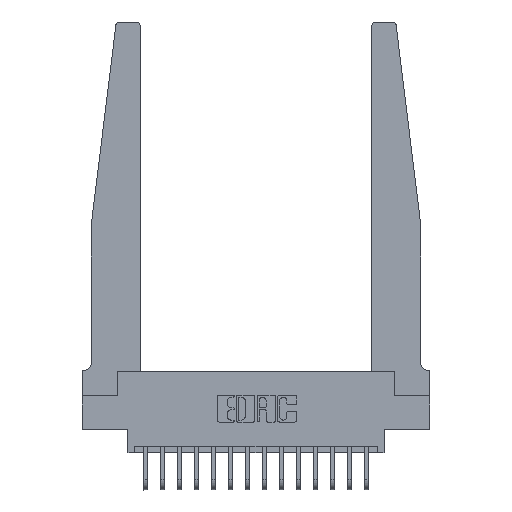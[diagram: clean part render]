
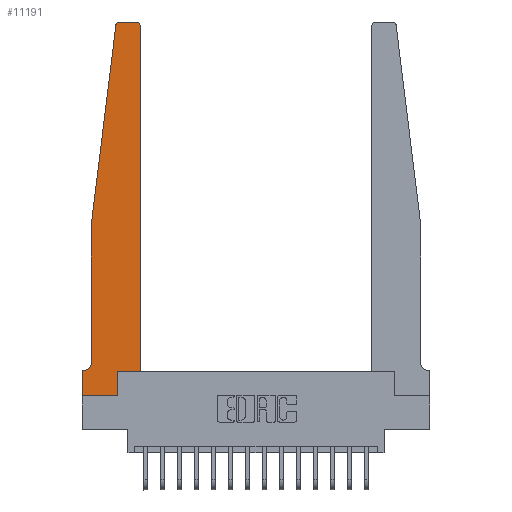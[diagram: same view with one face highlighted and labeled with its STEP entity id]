
A CAD part, top view. The second image highlights one B-rep face of the part: STEP entity #11191.
In plain terms, the highlighted planar face has unit normal (0, 0, 1).
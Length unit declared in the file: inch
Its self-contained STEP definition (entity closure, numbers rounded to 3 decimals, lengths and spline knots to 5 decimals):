
#123 = DIRECTION ( 'NONE',  ( 1., 0., 0. ) ) ;
#239 = CARTESIAN_POINT ( 'NONE',  ( 0.065, 0.2375, 0.37 ) ) ;
#549 = DIRECTION ( 'NONE',  ( -1., 0., 0. ) ) ;
#646 = DIRECTION ( 'NONE',  ( 0., 1., 0. ) ) ;
#913 = CARTESIAN_POINT ( 'NONE',  ( 0.425, 0.18, 0.37 ) ) ;
#951 = VERTEX_POINT ( 'NONE', #15004 ) ;
#1032 = DIRECTION ( 'NONE',  ( 0., 0., 1. ) ) ;
#1217 = PLANE ( 'NONE',  #14384 ) ;
#1465 = LINE ( 'NONE', #5619, #2724 ) ;
#1819 = DIRECTION ( 'NONE',  ( 0., -1., 0. ) ) ;
#1885 = VERTEX_POINT ( 'NONE', #15846 ) ;
#2092 = LINE ( 'NONE', #17278, #6125 ) ;
#2199 = EDGE_CURVE ( 'NONE', #13390, #1885, #1465, .T. ) ;
#2627 = VECTOR ( 'NONE', #4914, 39.37008 ) ;
#2724 = VECTOR ( 'NONE', #16654, 39.37008 ) ;
#2831 = DIRECTION ( 'NONE',  ( 0., 0., 1. ) ) ;
#2866 = VERTEX_POINT ( 'NONE', #12780 ) ;
#3019 = VERTEX_POINT ( 'NONE', #13405 ) ;
#3581 = ORIENTED_EDGE ( 'NONE', *, *, #2199, .T. ) ;
#3646 = VERTEX_POINT ( 'NONE', #12553 ) ;
#3770 = CARTESIAN_POINT ( 'NONE',  ( 0.065, 1.25, 0.37 ) ) ;
#3796 = EDGE_CURVE ( 'NONE', #3646, #10851, #15999, .T. ) ;
#3837 = CARTESIAN_POINT ( 'NONE',  ( 0., 0.1875, 0.37 ) ) ;
#3959 = EDGE_CURVE ( 'NONE', #10906, #951, #13307, .T. ) ;
#3970 = CIRCLE ( 'NONE', #7136, 0.03 ) ;
#4126 = VERTEX_POINT ( 'NONE', #15975 ) ;
#4410 = EDGE_CURVE ( 'NONE', #2866, #4126, #15384, .T. ) ;
#4660 = LINE ( 'NONE', #10174, #11518 ) ;
#4914 = DIRECTION ( 'NONE',  ( 0., 1., 0. ) ) ;
#4997 = EDGE_CURVE ( 'NONE', #4126, #16243, #14637, .T. ) ;
#5511 = AXIS2_PLACEMENT_3D ( 'NONE', #7934, #13445, #17621 ) ;
#5619 = CARTESIAN_POINT ( 'NONE',  ( 0., 0., 0.37 ) ) ;
#5694 = CIRCLE ( 'NONE', #9447, 0.03 ) ;
#5895 = DIRECTION ( 'NONE',  ( 0., 0., 1. ) ) ;
#6029 = ORIENTED_EDGE ( 'NONE', *, *, #12127, .T. ) ;
#6125 = VECTOR ( 'NONE', #1819, 39.37008 ) ;
#6710 = DIRECTION ( 'NONE',  ( 1., 0., 0. ) ) ;
#7136 = AXIS2_PLACEMENT_3D ( 'NONE', #17015, #5895, #11673 ) ;
#7484 = CARTESIAN_POINT ( 'NONE',  ( 0.25, 2.75, 0.37 ) ) ;
#7561 = VECTOR ( 'NONE', #14873, 39.37008 ) ;
#7923 = LINE ( 'NONE', #9371, #7561 ) ;
#7934 = CARTESIAN_POINT ( 'NONE',  ( 0.015, 0.2375, 0.37 ) ) ;
#8064 = EDGE_CURVE ( 'NONE', #10851, #11323, #5694, .T. ) ;
#8166 = EDGE_CURVE ( 'NONE', #16243, #3646, #3970, .T. ) ;
#8371 = CARTESIAN_POINT ( 'NONE',  ( 0., 0.1875, 0.37 ) ) ;
#8798 = DIRECTION ( 'NONE',  ( -1., 0., 0. ) ) ;
#9111 = VERTEX_POINT ( 'NONE', #3770 ) ;
#9371 = CARTESIAN_POINT ( 'NONE',  ( 0.065, 1.25, 0.37 ) ) ;
#9447 = AXIS2_PLACEMENT_3D ( 'NONE', #9781, #2831, #123 ) ;
#9781 = CARTESIAN_POINT ( 'NONE',  ( 0.27653, 2.72, 0.37 ) ) ;
#9873 = CARTESIAN_POINT ( 'NONE',  ( 0.425, 0.18, 0.37 ) ) ;
#9924 = ORIENTED_EDGE ( 'NONE', *, *, #4997, .T. ) ;
#10174 = CARTESIAN_POINT ( 'NONE',  ( 0., 0., 0.37 ) ) ;
#10181 = VECTOR ( 'NONE', #8798, 39.37008 ) ;
#10245 = LINE ( 'NONE', #13313, #2627 ) ;
#10266 = ORIENTED_EDGE ( 'NONE', *, *, #15518, .T. ) ;
#10301 = CARTESIAN_POINT ( 'NONE',  ( 0.24675, 2.72367, 0.37 ) ) ;
#10325 = CARTESIAN_POINT ( 'NONE',  ( 0.065, 0.1875, 0.37 ) ) ;
#10530 = EDGE_LOOP ( 'NONE', ( #11342, #16072, #14824, #10266, #12194, #12171, #3581, #6029, #13826, #17644, #9924, #15161 ) ) ;
#10851 = VERTEX_POINT ( 'NONE', #16953 ) ;
#10906 = VERTEX_POINT ( 'NONE', #239 ) ;
#11191 = ADVANCED_FACE ( 'NONE', ( #13752 ), #1217, .T. ) ;
#11323 = VERTEX_POINT ( 'NONE', #10301 ) ;
#11342 = ORIENTED_EDGE ( 'NONE', *, *, #3796, .T. ) ;
#11356 = VECTOR ( 'NONE', #646, 39.37008 ) ;
#11518 = VECTOR ( 'NONE', #15682, 39.37008 ) ;
#11673 = DIRECTION ( 'NONE',  ( 1., 0., 0. ) ) ;
#12127 = EDGE_CURVE ( 'NONE', #1885, #3019, #4660, .T. ) ;
#12171 = ORIENTED_EDGE ( 'NONE', *, *, #17859, .T. ) ;
#12194 = ORIENTED_EDGE ( 'NONE', *, *, #3959, .T. ) ;
#12553 = CARTESIAN_POINT ( 'NONE',  ( 0.395, 2.75, 0.37 ) ) ;
#12581 = DIRECTION ( 'NONE',  ( 1., 0., 0. ) ) ;
#12780 = CARTESIAN_POINT ( 'NONE',  ( 0.2605, 0.18, 0.37 ) ) ;
#13307 = CIRCLE ( 'NONE', #5511, 0.05 ) ;
#13313 = CARTESIAN_POINT ( 'NONE',  ( 0.2605, 0.18, 0.37 ) ) ;
#13390 = VERTEX_POINT ( 'NONE', #8371 ) ;
#13405 = CARTESIAN_POINT ( 'NONE',  ( 0.2605, 0., 0.37 ) ) ;
#13445 = DIRECTION ( 'NONE',  ( 0., 0., -1. ) ) ;
#13752 = FACE_OUTER_BOUND ( 'NONE', #10530, .T. ) ;
#13826 = ORIENTED_EDGE ( 'NONE', *, *, #16228, .T. ) ;
#14384 = AXIS2_PLACEMENT_3D ( 'NONE', #3837, #1032, #6710 ) ;
#14499 = CARTESIAN_POINT ( 'NONE',  ( 0.425, 2.72, 0.37 ) ) ;
#14637 = LINE ( 'NONE', #913, #11356 ) ;
#14824 = ORIENTED_EDGE ( 'NONE', *, *, #17061, .T. ) ;
#14873 = DIRECTION ( 'NONE',  ( -0.122, -0.992, 0. ) ) ;
#15004 = CARTESIAN_POINT ( 'NONE',  ( 0.015, 0.1875, 0.37 ) ) ;
#15068 = VECTOR ( 'NONE', #549, 39.37008 ) ;
#15161 = ORIENTED_EDGE ( 'NONE', *, *, #8166, .T. ) ;
#15384 = LINE ( 'NONE', #9873, #15669 ) ;
#15518 = EDGE_CURVE ( 'NONE', #9111, #10906, #2092, .T. ) ;
#15669 = VECTOR ( 'NONE', #12581, 39.37008 ) ;
#15682 = DIRECTION ( 'NONE',  ( 1., 0., 0. ) ) ;
#15846 = CARTESIAN_POINT ( 'NONE',  ( 0., 0., 0.37 ) ) ;
#15975 = CARTESIAN_POINT ( 'NONE',  ( 0.425, 0.18, 0.37 ) ) ;
#15999 = LINE ( 'NONE', #7484, #15068 ) ;
#16072 = ORIENTED_EDGE ( 'NONE', *, *, #8064, .T. ) ;
#16228 = EDGE_CURVE ( 'NONE', #3019, #2866, #10245, .T. ) ;
#16243 = VERTEX_POINT ( 'NONE', #14499 ) ;
#16654 = DIRECTION ( 'NONE',  ( 0., -1., 0. ) ) ;
#16953 = CARTESIAN_POINT ( 'NONE',  ( 0.27653, 2.75, 0.37 ) ) ;
#17015 = CARTESIAN_POINT ( 'NONE',  ( 0.395, 2.72, 0.37 ) ) ;
#17061 = EDGE_CURVE ( 'NONE', #11323, #9111, #7923, .T. ) ;
#17204 = LINE ( 'NONE', #10325, #10181 ) ;
#17278 = CARTESIAN_POINT ( 'NONE',  ( 0.065, 1.25, 0.37 ) ) ;
#17621 = DIRECTION ( 'NONE',  ( -1., 0., 0. ) ) ;
#17644 = ORIENTED_EDGE ( 'NONE', *, *, #4410, .T. ) ;
#17859 = EDGE_CURVE ( 'NONE', #951, #13390, #17204, .T. ) ;
